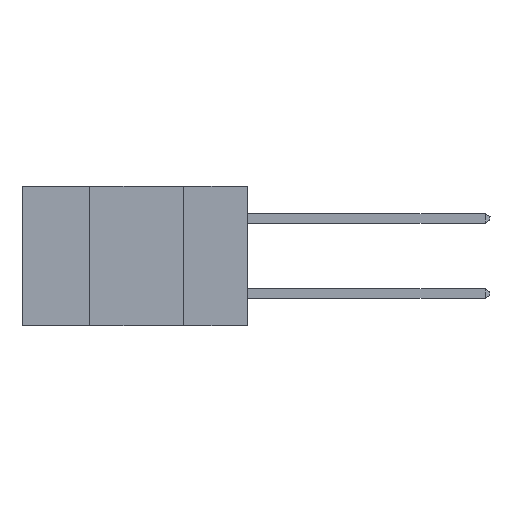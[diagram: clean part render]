
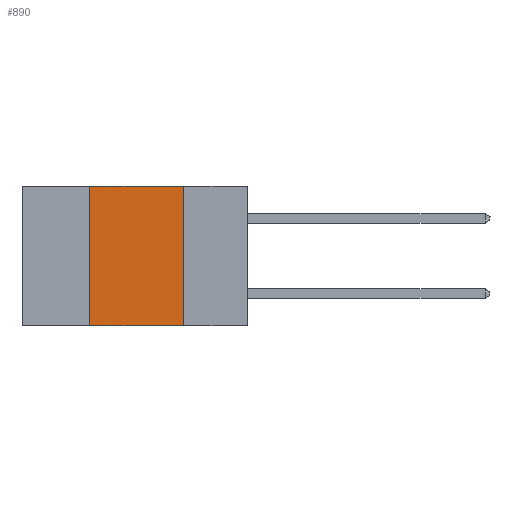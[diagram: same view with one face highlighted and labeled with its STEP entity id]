
A CAD part, left-side view. The second image highlights one B-rep face of the part: STEP entity #890.
In plain terms, the highlighted planar face has unit normal (-1, 0, 0).
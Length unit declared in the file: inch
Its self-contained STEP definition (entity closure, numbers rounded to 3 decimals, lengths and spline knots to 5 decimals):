
#890 = ADVANCED_FACE ( 'NONE', ( #18095 ), #12822, .F. ) ;
#1076 = LINE ( 'NONE', #4856, #16607 ) ;
#2938 = EDGE_CURVE ( 'NONE', #11536, #19067, #1076, .T. ) ;
#3181 = DIRECTION ( 'NONE',  ( 0., 0., -1. ) ) ;
#3277 = ORIENTED_EDGE ( 'NONE', *, *, #21834, .T. ) ;
#4015 = LINE ( 'NONE', #7664, #20246 ) ;
#4856 = CARTESIAN_POINT ( 'NONE',  ( 0., 0.17, -0.37 ) ) ;
#5377 = VERTEX_POINT ( 'NONE', #6875 ) ;
#5885 = DIRECTION ( 'NONE',  ( 0., 0., 1. ) ) ;
#6003 = LINE ( 'NONE', #22004, #19361 ) ;
#6875 = CARTESIAN_POINT ( 'NONE',  ( 0., 0.42, -0.37 ) ) ;
#7114 = AXIS2_PLACEMENT_3D ( 'NONE', #12939, #11287, #18221 ) ;
#7306 = ORIENTED_EDGE ( 'NONE', *, *, #19107, .F. ) ;
#7664 = CARTESIAN_POINT ( 'NONE',  ( 0., 0.6, 0. ) ) ;
#7704 = DIRECTION ( 'NONE',  ( 0., -1., 0. ) ) ;
#8438 = VERTEX_POINT ( 'NONE', #22307 ) ;
#9701 = CARTESIAN_POINT ( 'NONE',  ( 0., 0.6, -0.37 ) ) ;
#10059 = ORIENTED_EDGE ( 'NONE', *, *, #2938, .F. ) ;
#10403 = CARTESIAN_POINT ( 'NONE',  ( 0., 0.17, 0. ) ) ;
#11287 = DIRECTION ( 'NONE',  ( 1., 0., 0. ) ) ;
#11536 = VERTEX_POINT ( 'NONE', #10403 ) ;
#12759 = LINE ( 'NONE', #9701, #15428 ) ;
#12822 = PLANE ( 'NONE',  #7114 ) ;
#12939 = CARTESIAN_POINT ( 'NONE',  ( 0., 0.6, 0. ) ) ;
#12993 = EDGE_LOOP ( 'NONE', ( #10059, #7306, #15229, #3277 ) ) ;
#13188 = CARTESIAN_POINT ( 'NONE',  ( 0., 0.17, -0.37 ) ) ;
#13416 = DIRECTION ( 'NONE',  ( 0., -1., 0. ) ) ;
#14120 = EDGE_CURVE ( 'NONE', #5377, #8438, #6003, .T. ) ;
#15229 = ORIENTED_EDGE ( 'NONE', *, *, #14120, .F. ) ;
#15428 = VECTOR ( 'NONE', #7704, 39.37008 ) ;
#16607 = VECTOR ( 'NONE', #3181, 39.37008 ) ;
#18095 = FACE_OUTER_BOUND ( 'NONE', #12993, .T. ) ;
#18221 = DIRECTION ( 'NONE',  ( 0., 0., -1. ) ) ;
#19067 = VERTEX_POINT ( 'NONE', #13188 ) ;
#19107 = EDGE_CURVE ( 'NONE', #8438, #11536, #4015, .T. ) ;
#19361 = VECTOR ( 'NONE', #5885, 39.37008 ) ;
#20246 = VECTOR ( 'NONE', #13416, 39.37008 ) ;
#21834 = EDGE_CURVE ( 'NONE', #5377, #19067, #12759, .T. ) ;
#22004 = CARTESIAN_POINT ( 'NONE',  ( 0., 0.42, -0.37 ) ) ;
#22307 = CARTESIAN_POINT ( 'NONE',  ( 0., 0.42, 0. ) ) ;
